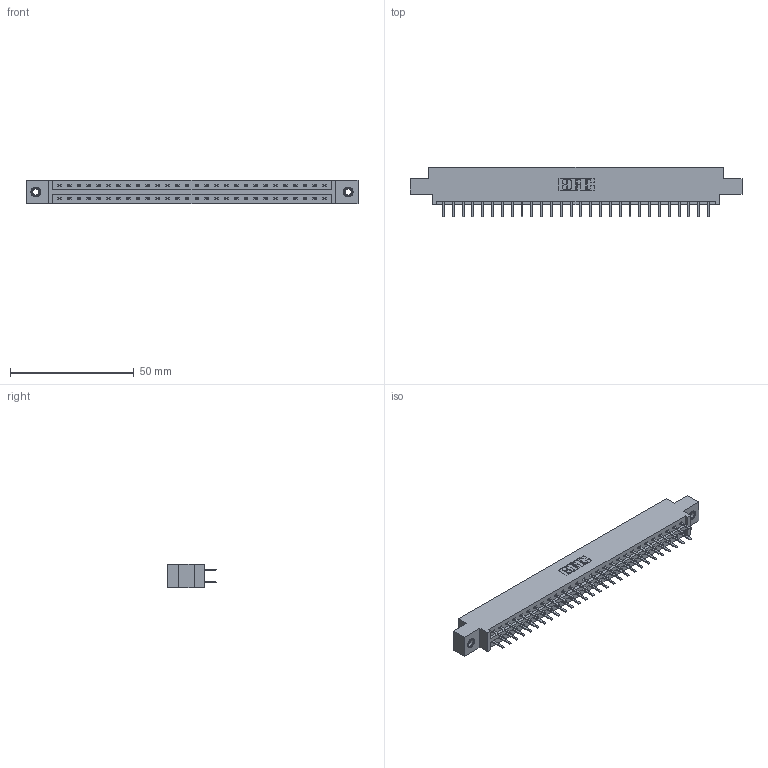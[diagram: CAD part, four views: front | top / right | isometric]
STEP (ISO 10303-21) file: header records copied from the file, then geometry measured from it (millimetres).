
FILE_DESCRIPTION (( 'STEP AP203' ), '1' );
FILE_NAME ('337-056-520-807.STEP', '2019-10-11T19:33:51', ( '' ), ( '' ), 'SwSTEP 2.0', 'SolidWorks 2016', '' );
FILE_SCHEMA (( 'CONFIG_CONTROL_DESIGN' ));
Length unit declared in the file: inch
Products named in the file (4): 345-292-001_345-293-120; 337-056-520-807; 337 Part_0.170 Offset - 0.156 Dia-TI; 345-250-001_345-250-005-103
Assembly tree (59 placements, depth 2):
  337-056-520-807
    337 Part_0.170 Offset - 0.156 Dia-TI
    345-292-001_345-293-120  x56
    345-250-001_345-250-005-103  x2
Bounding box: 133.96 x 20.02 x 9.4 mm (x, y, z)
Volume: 13775.7 mm3; surface area: 15511.1 mm2
Topology: 59 solids, 59 shells, 3426 faces, 9923 edges, 6458 vertices
Faces by surface type: plane 2346, cylinder 1064, cone 12, torus 4
Entity records: 24952 total; most frequent: CARTESIAN_POINT 4209, ORIENTED_EDGE 4126, DIRECTION 3625, EDGE_CURVE 2063, LINE 1911, VECTOR 1911, VERTEX_POINT 1368, AXIS2_PLACEMENT_3D 857
